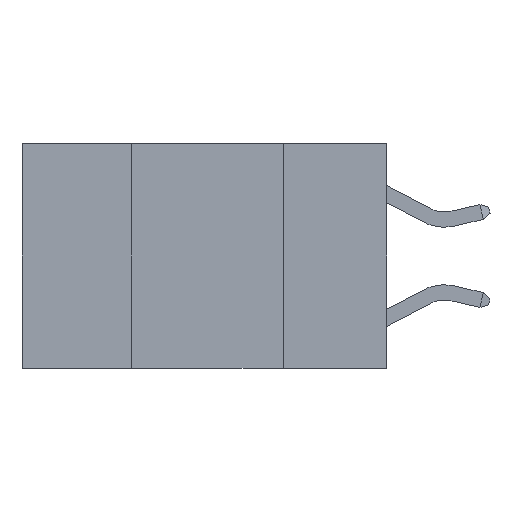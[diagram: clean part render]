
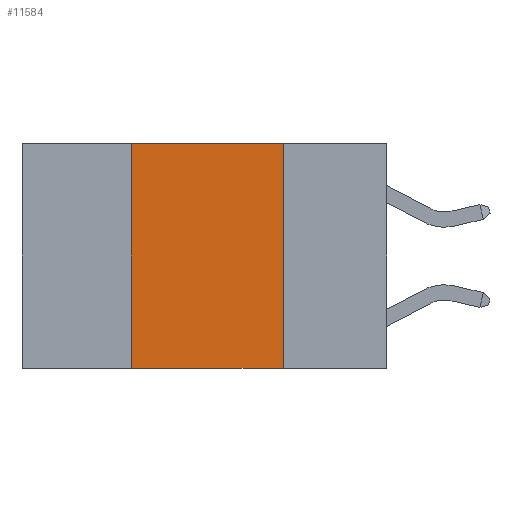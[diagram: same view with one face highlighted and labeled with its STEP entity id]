
A CAD part, left-side view. The second image highlights one B-rep face of the part: STEP entity #11584.
In plain terms, the highlighted planar face has unit normal (-1, 0, 0).
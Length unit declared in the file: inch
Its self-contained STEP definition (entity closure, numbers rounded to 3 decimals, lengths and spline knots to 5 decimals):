
#2473 = DIRECTION ( 'NONE',  ( 0., 0., -1. ) ) ;
#2842 = VECTOR ( 'NONE', #4342, 39.37008 ) ;
#4342 = DIRECTION ( 'NONE',  ( 0., -1., 0. ) ) ;
#4779 = ORIENTED_EDGE ( 'NONE', *, *, #9531, .F. ) ;
#6729 = EDGE_CURVE ( 'NONE', #17543, #23409, #15551, .T. ) ;
#7369 = CARTESIAN_POINT ( 'NONE',  ( 0., 0.6, 0. ) ) ;
#8243 = LINE ( 'NONE', #17640, #19618 ) ;
#8531 = CARTESIAN_POINT ( 'NONE',  ( 0., 0.6, -0.37 ) ) ;
#9479 = ORIENTED_EDGE ( 'NONE', *, *, #6729, .F. ) ;
#9531 = EDGE_CURVE ( 'NONE', #9928, #17543, #12673, .T. ) ;
#9928 = VERTEX_POINT ( 'NONE', #24582 ) ;
#11034 = ORIENTED_EDGE ( 'NONE', *, *, #22945, .F. ) ;
#11045 = VERTEX_POINT ( 'NONE', #11881 ) ;
#11584 = ADVANCED_FACE ( 'NONE', ( #24781 ), #20836, .F. ) ;
#11881 = CARTESIAN_POINT ( 'NONE',  ( 0., 0.42, -0.37 ) ) ;
#12673 = LINE ( 'NONE', #20902, #20101 ) ;
#13834 = DIRECTION ( 'NONE',  ( 0., 0., 1. ) ) ;
#14337 = DIRECTION ( 'NONE',  ( 0., -1., 0. ) ) ;
#14879 = CARTESIAN_POINT ( 'NONE',  ( 0., 0.17, 0. ) ) ;
#15551 = LINE ( 'NONE', #17714, #17290 ) ;
#16056 = EDGE_CURVE ( 'NONE', #11045, #23409, #20199, .T. ) ;
#17242 = DIRECTION ( 'NONE',  ( 0., 0., -1. ) ) ;
#17290 = VECTOR ( 'NONE', #2473, 39.37008 ) ;
#17543 = VERTEX_POINT ( 'NONE', #14879 ) ;
#17640 = CARTESIAN_POINT ( 'NONE',  ( 0., 0.42, 0. ) ) ;
#17714 = CARTESIAN_POINT ( 'NONE',  ( 0., 0.17, 0. ) ) ;
#19618 = VECTOR ( 'NONE', #13834, 39.37008 ) ;
#20101 = VECTOR ( 'NONE', #14337, 39.37008 ) ;
#20199 = LINE ( 'NONE', #8531, #2842 ) ;
#20836 = PLANE ( 'NONE',  #21814 ) ;
#20902 = CARTESIAN_POINT ( 'NONE',  ( 0., 0.6, 0. ) ) ;
#21700 = CARTESIAN_POINT ( 'NONE',  ( 0., 0.17, -0.37 ) ) ;
#21814 = AXIS2_PLACEMENT_3D ( 'NONE', #7369, #24908, #17242 ) ;
#22567 = ORIENTED_EDGE ( 'NONE', *, *, #16056, .T. ) ;
#22945 = EDGE_CURVE ( 'NONE', #11045, #9928, #8243, .T. ) ;
#23130 = EDGE_LOOP ( 'NONE', ( #9479, #4779, #11034, #22567 ) ) ;
#23409 = VERTEX_POINT ( 'NONE', #21700 ) ;
#24582 = CARTESIAN_POINT ( 'NONE',  ( 0., 0.42, 0. ) ) ;
#24781 = FACE_OUTER_BOUND ( 'NONE', #23130, .T. ) ;
#24908 = DIRECTION ( 'NONE',  ( 1., 0., 0. ) ) ;
